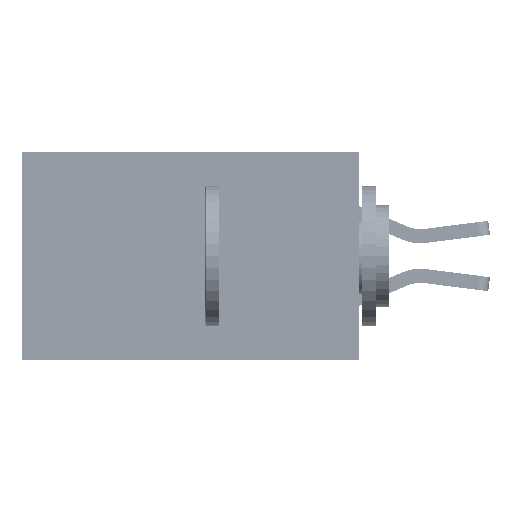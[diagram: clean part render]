
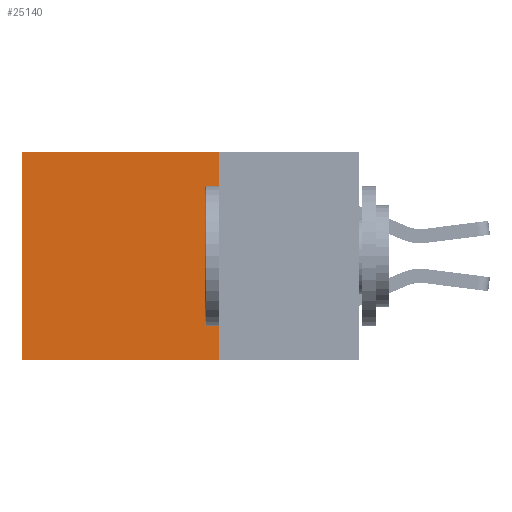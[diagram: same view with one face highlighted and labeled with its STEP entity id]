
A CAD part, left-side view. The second image highlights one B-rep face of the part: STEP entity #25140.
In plain terms, the highlighted planar face has unit normal (-1, 0, 0).
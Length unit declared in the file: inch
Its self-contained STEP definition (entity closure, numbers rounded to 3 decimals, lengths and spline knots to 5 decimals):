
#363 = PLANE ( 'NONE',  #36069 ) ;
#979 = VERTEX_POINT ( 'NONE', #22802 ) ;
#1254 = CARTESIAN_POINT ( 'NONE',  ( 0.2875, 0.25, 0. ) ) ;
#3112 = FACE_OUTER_BOUND ( 'NONE', #35848, .T. ) ;
#4050 = DIRECTION ( 'NONE',  ( 0., 0., -1. ) ) ;
#4430 = VECTOR ( 'NONE', #10824, 39.37008 ) ;
#4924 = EDGE_CURVE ( 'NONE', #979, #22922, #27832, .T. ) ;
#6042 = ORIENTED_EDGE ( 'NONE', *, *, #28372, .T. ) ;
#7122 = DIRECTION ( 'NONE',  ( 0., 1., 0. ) ) ;
#7508 = CARTESIAN_POINT ( 'NONE',  ( 0.2875, 0.25, 0. ) ) ;
#9318 = ORIENTED_EDGE ( 'NONE', *, *, #42226, .F. ) ;
#10758 = CARTESIAN_POINT ( 'NONE',  ( 0.2875, 0.25, 0. ) ) ;
#10824 = DIRECTION ( 'NONE',  ( 0., 1., 0. ) ) ;
#16680 = CARTESIAN_POINT ( 'NONE',  ( 0.2875, 0.25, -0.37 ) ) ;
#19245 = CARTESIAN_POINT ( 'NONE',  ( 0.2875, 0.6, 0. ) ) ;
#19616 = LINE ( 'NONE', #7508, #42047 ) ;
#21062 = CARTESIAN_POINT ( 'NONE',  ( 0.2875, 0.6, 0. ) ) ;
#22112 = EDGE_CURVE ( 'NONE', #34906, #36128, #31353, .T. ) ;
#22375 = VECTOR ( 'NONE', #4050, 39.37008 ) ;
#22802 = CARTESIAN_POINT ( 'NONE',  ( 0.2875, 0.25, 0. ) ) ;
#22922 = VERTEX_POINT ( 'NONE', #19245 ) ;
#24295 = CARTESIAN_POINT ( 'NONE',  ( 0.2875, 0.25, -0.37 ) ) ;
#24863 = ORIENTED_EDGE ( 'NONE', *, *, #22112, .F. ) ;
#24899 = DIRECTION ( 'NONE',  ( 0., 0., -1. ) ) ;
#25140 = ADVANCED_FACE ( 'NONE', ( #3112 ), #363, .F. ) ;
#26608 = ORIENTED_EDGE ( 'NONE', *, *, #4924, .T. ) ;
#27401 = CARTESIAN_POINT ( 'NONE',  ( 0.2875, 0.6, -0.37 ) ) ;
#27832 = LINE ( 'NONE', #1254, #28893 ) ;
#28372 = EDGE_CURVE ( 'NONE', #22922, #36128, #36810, .T. ) ;
#28893 = VECTOR ( 'NONE', #7122, 39.37008 ) ;
#31353 = LINE ( 'NONE', #16680, #4430 ) ;
#34897 = DIRECTION ( 'NONE',  ( 1., 0., 0. ) ) ;
#34906 = VERTEX_POINT ( 'NONE', #24295 ) ;
#35848 = EDGE_LOOP ( 'NONE', ( #6042, #24863, #9318, #26608 ) ) ;
#36069 = AXIS2_PLACEMENT_3D ( 'NONE', #10758, #34897, #24899 ) ;
#36128 = VERTEX_POINT ( 'NONE', #27401 ) ;
#36810 = LINE ( 'NONE', #21062, #22375 ) ;
#41635 = DIRECTION ( 'NONE',  ( 0., 0., -1. ) ) ;
#42047 = VECTOR ( 'NONE', #41635, 39.37008 ) ;
#42226 = EDGE_CURVE ( 'NONE', #979, #34906, #19616, .T. ) ;
